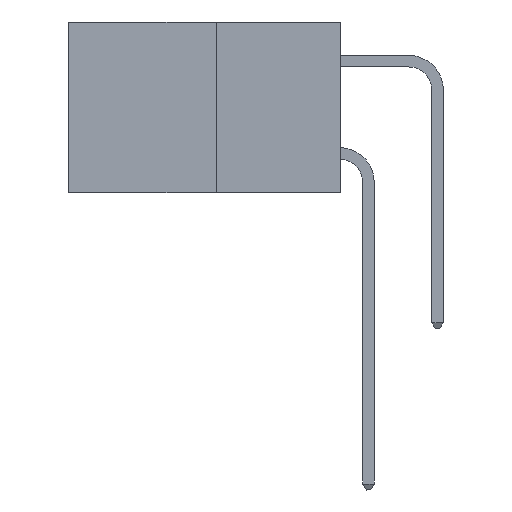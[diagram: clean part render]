
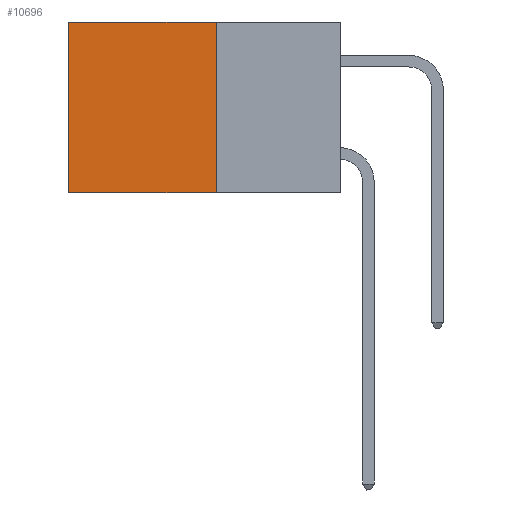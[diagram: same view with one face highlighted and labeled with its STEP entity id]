
A CAD part, left-side view. The second image highlights one B-rep face of the part: STEP entity #10696.
In plain terms, the highlighted planar face has unit normal (-1, 0, 0).
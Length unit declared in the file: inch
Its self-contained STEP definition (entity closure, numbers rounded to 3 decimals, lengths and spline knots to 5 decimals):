
#939 = VERTEX_POINT ( 'NONE', #16175 ) ;
#1692 = DIRECTION ( 'NONE',  ( 0., 0., -1. ) ) ;
#1812 = CARTESIAN_POINT ( 'NONE',  ( 0.277, 0.59, -0.37 ) ) ;
#3136 = LINE ( 'NONE', #7919, #7535 ) ;
#3203 = VECTOR ( 'NONE', #1692, 39.37008 ) ;
#3262 = DIRECTION ( 'NONE',  ( 0., 0., -1. ) ) ;
#3267 = CARTESIAN_POINT ( 'NONE',  ( 0.277, 0.27, -0.37 ) ) ;
#5511 = VECTOR ( 'NONE', #3262, 39.37008 ) ;
#5761 = VERTEX_POINT ( 'NONE', #16163 ) ;
#6253 = ORIENTED_EDGE ( 'NONE', *, *, #15873, .F. ) ;
#6359 = EDGE_CURVE ( 'NONE', #15914, #939, #19908, .T. ) ;
#6468 = EDGE_CURVE ( 'NONE', #5761, #13544, #9394, .T. ) ;
#6899 = CARTESIAN_POINT ( 'NONE',  ( 0.277, 0.27, -0.37 ) ) ;
#7535 = VECTOR ( 'NONE', #15978, 39.37008 ) ;
#7919 = CARTESIAN_POINT ( 'NONE',  ( 0.277, 0.27, -0.37 ) ) ;
#8481 = ORIENTED_EDGE ( 'NONE', *, *, #8998, .T. ) ;
#8998 = EDGE_CURVE ( 'NONE', #5761, #15914, #14651, .T. ) ;
#9376 = DIRECTION ( 'NONE',  ( 0., 1., 0. ) ) ;
#9394 = LINE ( 'NONE', #3267, #5511 ) ;
#9496 = CARTESIAN_POINT ( 'NONE',  ( 0.277, 0.27, 0. ) ) ;
#10696 = ADVANCED_FACE ( 'NONE', ( #15847 ), #19850, .F. ) ;
#11234 = CARTESIAN_POINT ( 'NONE',  ( 0.277, 0.59, 0. ) ) ;
#11890 = AXIS2_PLACEMENT_3D ( 'NONE', #19607, #19582, #19519 ) ;
#12670 = ORIENTED_EDGE ( 'NONE', *, *, #6468, .F. ) ;
#13544 = VERTEX_POINT ( 'NONE', #6899 ) ;
#14651 = LINE ( 'NONE', #9496, #15143 ) ;
#15143 = VECTOR ( 'NONE', #9376, 39.37008 ) ;
#15800 = ORIENTED_EDGE ( 'NONE', *, *, #6359, .T. ) ;
#15847 = FACE_OUTER_BOUND ( 'NONE', #15890, .T. ) ;
#15873 = EDGE_CURVE ( 'NONE', #13544, #939, #3136, .T. ) ;
#15890 = EDGE_LOOP ( 'NONE', ( #15800, #6253, #12670, #8481 ) ) ;
#15914 = VERTEX_POINT ( 'NONE', #11234 ) ;
#15978 = DIRECTION ( 'NONE',  ( 0., 1., 0. ) ) ;
#16163 = CARTESIAN_POINT ( 'NONE',  ( 0.277, 0.27, 0. ) ) ;
#16175 = CARTESIAN_POINT ( 'NONE',  ( 0.277, 0.59, -0.37 ) ) ;
#19519 = DIRECTION ( 'NONE',  ( 0., 0., -1. ) ) ;
#19582 = DIRECTION ( 'NONE',  ( 1., 0., 0. ) ) ;
#19607 = CARTESIAN_POINT ( 'NONE',  ( 0.277, 0.27, -0.37 ) ) ;
#19850 = PLANE ( 'NONE',  #11890 ) ;
#19908 = LINE ( 'NONE', #1812, #3203 ) ;
